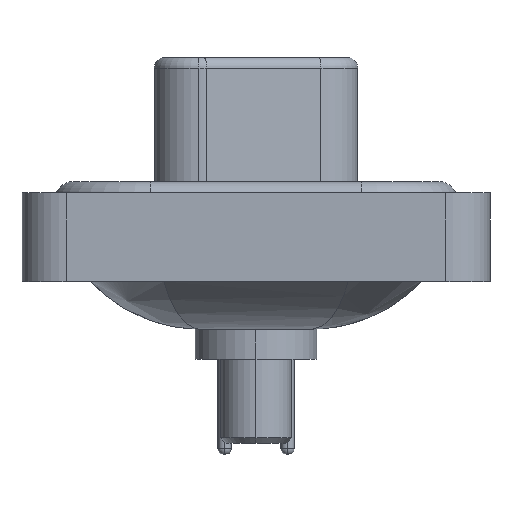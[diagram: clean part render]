
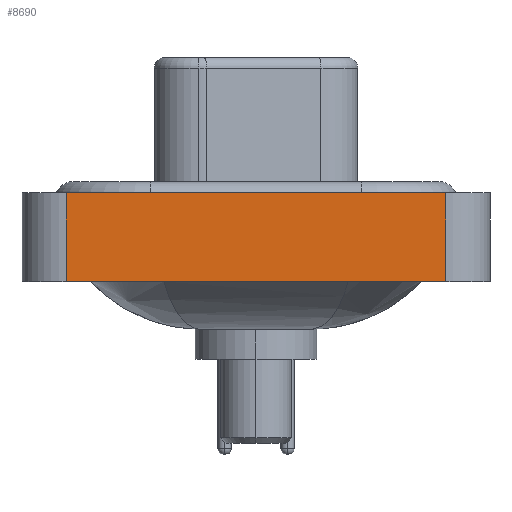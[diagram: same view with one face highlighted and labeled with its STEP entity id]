
A CAD part, left-side view. The second image highlights one B-rep face of the part: STEP entity #8690.
In plain terms, the highlighted planar face has unit normal (-1, 0, 0).
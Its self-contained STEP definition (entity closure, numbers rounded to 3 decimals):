
#911 = AXIS2_PLACEMENT_3D ( 'NONE', #5037, #2203, #14151 ) ;
#1672 = VERTEX_POINT ( 'NONE', #12767 ) ;
#1775 = EDGE_CURVE ( 'NONE', #4312, #8124, #15289, .T. ) ;
#2203 = DIRECTION ( 'NONE',  ( -1., 0., 0. ) ) ;
#2391 = PLANE ( 'NONE',  #911 ) ;
#2436 = VECTOR ( 'NONE', #5381, 1000. ) ;
#2613 = EDGE_CURVE ( 'NONE', #16026, #1672, #10717, .T. ) ;
#3524 = CARTESIAN_POINT ( 'NONE',  ( -7.3, -8.55, -3.6 ) ) ;
#3609 = EDGE_CURVE ( 'NONE', #1672, #8124, #6196, .T. ) ;
#4312 = VERTEX_POINT ( 'NONE', #3524 ) ;
#4457 = ORIENTED_EDGE ( 'NONE', *, *, #1775, .T. ) ;
#5037 = CARTESIAN_POINT ( 'NONE',  ( -7.3, -8.55, -3.6 ) ) ;
#5273 = VECTOR ( 'NONE', #9375, 1000. ) ;
#5279 = LINE ( 'NONE', #9748, #10885 ) ;
#5381 = DIRECTION ( 'NONE',  ( 0., 0., 1. ) ) ;
#5471 = DIRECTION ( 'NONE',  ( 0., -1., 0. ) ) ;
#6168 = CARTESIAN_POINT ( 'NONE',  ( -7.3, 8.55, -3.6 ) ) ;
#6196 = LINE ( 'NONE', #16647, #15421 ) ;
#7763 = DIRECTION ( 'NONE',  ( 0., -1., 0. ) ) ;
#8124 = VERTEX_POINT ( 'NONE', #11954 ) ;
#8690 = ADVANCED_FACE ( 'NONE', ( #15601 ), #2391, .T. ) ;
#9375 = DIRECTION ( 'NONE',  ( 0., 0., 1. ) ) ;
#9748 = CARTESIAN_POINT ( 'NONE',  ( -7.3, -8.55, -3.6 ) ) ;
#9774 = EDGE_LOOP ( 'NONE', ( #4457, #12979, #11852, #12063 ) ) ;
#10717 = LINE ( 'NONE', #13736, #5273 ) ;
#10885 = VECTOR ( 'NONE', #5471, 1000. ) ;
#11050 = EDGE_CURVE ( 'NONE', #16026, #4312, #5279, .T. ) ;
#11852 = ORIENTED_EDGE ( 'NONE', *, *, #2613, .F. ) ;
#11954 = CARTESIAN_POINT ( 'NONE',  ( -7.3, -8.55, 0.4 ) ) ;
#12063 = ORIENTED_EDGE ( 'NONE', *, *, #11050, .T. ) ;
#12767 = CARTESIAN_POINT ( 'NONE',  ( -7.3, 8.55, 0.4 ) ) ;
#12979 = ORIENTED_EDGE ( 'NONE', *, *, #3609, .F. ) ;
#13736 = CARTESIAN_POINT ( 'NONE',  ( -7.3, 8.55, -3.6 ) ) ;
#14151 = DIRECTION ( 'NONE',  ( 0., 0., 1. ) ) ;
#15289 = LINE ( 'NONE', #18678, #2436 ) ;
#15421 = VECTOR ( 'NONE', #7763, 1000. ) ;
#15601 = FACE_OUTER_BOUND ( 'NONE', #9774, .T. ) ;
#16026 = VERTEX_POINT ( 'NONE', #6168 ) ;
#16647 = CARTESIAN_POINT ( 'NONE',  ( -7.3, -8.55, 0.4 ) ) ;
#18678 = CARTESIAN_POINT ( 'NONE',  ( -7.3, -8.55, -3.6 ) ) ;
